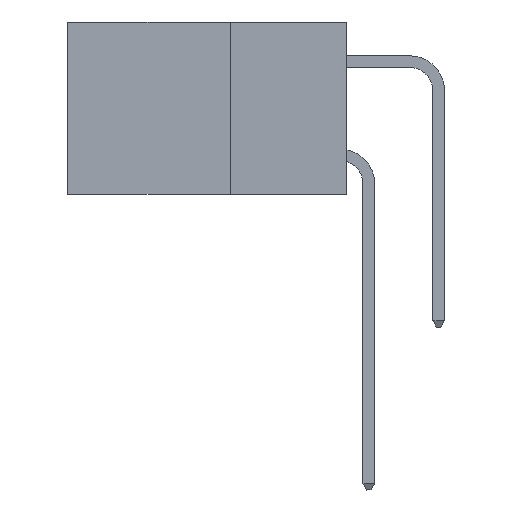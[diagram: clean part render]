
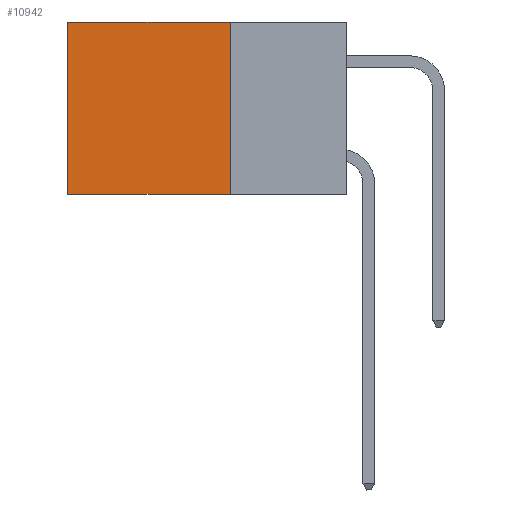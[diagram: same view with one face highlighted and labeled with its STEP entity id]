
A CAD part, left-side view. The second image highlights one B-rep face of the part: STEP entity #10942.
In plain terms, the highlighted planar face has unit normal (-1, 0, 0).
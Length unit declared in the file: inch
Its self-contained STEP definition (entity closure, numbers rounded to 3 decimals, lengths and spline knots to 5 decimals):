
#58 = LINE ( 'NONE', #15202, #14516 ) ;
#2323 = DIRECTION ( 'NONE',  ( 1., 0., 0. ) ) ;
#2439 = EDGE_CURVE ( 'NONE', #15430, #2598, #7643, .T. ) ;
#2598 = VERTEX_POINT ( 'NONE', #18295 ) ;
#4860 = DIRECTION ( 'NONE',  ( 0., 1., 0. ) ) ;
#5759 = VECTOR ( 'NONE', #10868, 39.37008 ) ;
#5798 = VECTOR ( 'NONE', #9021, 39.37008 ) ;
#6170 = EDGE_LOOP ( 'NONE', ( #7955, #14919, #14326, #18561 ) ) ;
#6359 = VERTEX_POINT ( 'NONE', #12972 ) ;
#7643 = LINE ( 'NONE', #14907, #19844 ) ;
#7955 = ORIENTED_EDGE ( 'NONE', *, *, #14308, .T. ) ;
#8119 = CARTESIAN_POINT ( 'NONE',  ( 0.2875, 0.6, -0.37 ) ) ;
#9021 = DIRECTION ( 'NONE',  ( 0., 1., 0. ) ) ;
#9743 = PLANE ( 'NONE',  #12024 ) ;
#9758 = FACE_OUTER_BOUND ( 'NONE', #6170, .T. ) ;
#10424 = LINE ( 'NONE', #15145, #5798 ) ;
#10868 = DIRECTION ( 'NONE',  ( 0., 0., -1. ) ) ;
#10942 = ADVANCED_FACE ( 'NONE', ( #9758 ), #9743, .F. ) ;
#11665 = CARTESIAN_POINT ( 'NONE',  ( 0.2875, 0.25, 0. ) ) ;
#12024 = AXIS2_PLACEMENT_3D ( 'NONE', #11665, #2323, #14210 ) ;
#12160 = CARTESIAN_POINT ( 'NONE',  ( 0.2875, 0.6, 0. ) ) ;
#12972 = CARTESIAN_POINT ( 'NONE',  ( 0.2875, 0.6, 0. ) ) ;
#13085 = LINE ( 'NONE', #12160, #5759 ) ;
#14210 = DIRECTION ( 'NONE',  ( 0., 0., -1. ) ) ;
#14308 = EDGE_CURVE ( 'NONE', #6359, #20013, #13085, .T. ) ;
#14326 = ORIENTED_EDGE ( 'NONE', *, *, #2439, .F. ) ;
#14516 = VECTOR ( 'NONE', #4860, 39.37008 ) ;
#14523 = EDGE_CURVE ( 'NONE', #15430, #6359, #58, .T. ) ;
#14907 = CARTESIAN_POINT ( 'NONE',  ( 0.2875, 0.25, 0. ) ) ;
#14919 = ORIENTED_EDGE ( 'NONE', *, *, #19716, .F. ) ;
#15145 = CARTESIAN_POINT ( 'NONE',  ( 0.2875, 0.25, -0.37 ) ) ;
#15202 = CARTESIAN_POINT ( 'NONE',  ( 0.2875, 0.25, 0. ) ) ;
#15430 = VERTEX_POINT ( 'NONE', #20087 ) ;
#16402 = DIRECTION ( 'NONE',  ( 0., 0., -1. ) ) ;
#18295 = CARTESIAN_POINT ( 'NONE',  ( 0.2875, 0.25, -0.37 ) ) ;
#18561 = ORIENTED_EDGE ( 'NONE', *, *, #14523, .T. ) ;
#19716 = EDGE_CURVE ( 'NONE', #2598, #20013, #10424, .T. ) ;
#19844 = VECTOR ( 'NONE', #16402, 39.37008 ) ;
#20013 = VERTEX_POINT ( 'NONE', #8119 ) ;
#20087 = CARTESIAN_POINT ( 'NONE',  ( 0.2875, 0.25, 0. ) ) ;
